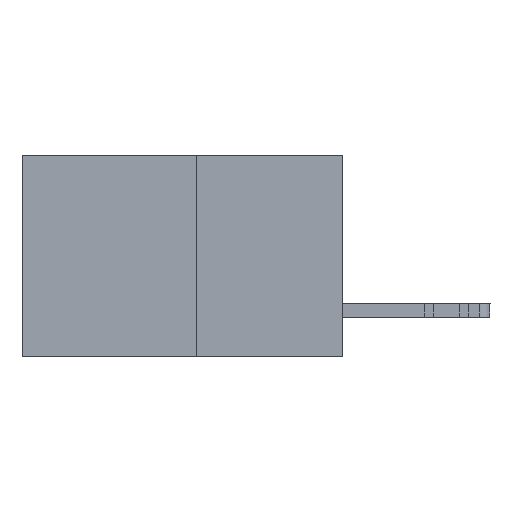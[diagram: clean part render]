
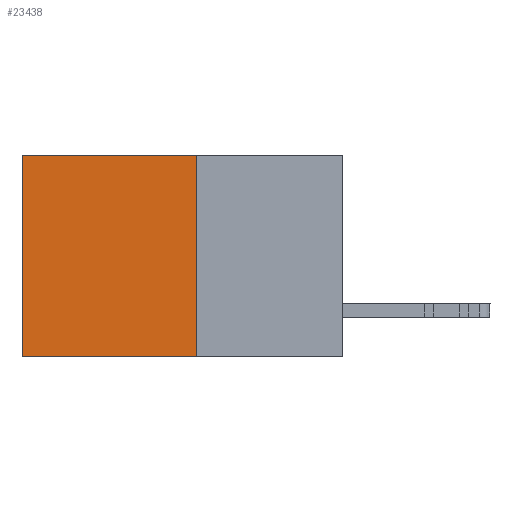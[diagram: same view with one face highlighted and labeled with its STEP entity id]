
A CAD part, left-side view. The second image highlights one B-rep face of the part: STEP entity #23438.
In plain terms, the highlighted planar face has unit normal (-1, 0, 0).
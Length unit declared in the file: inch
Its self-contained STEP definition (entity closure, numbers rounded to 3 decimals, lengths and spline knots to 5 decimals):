
#1456 = EDGE_CURVE ( 'NONE', #12765, #17585, #30709, .T. ) ;
#2441 = LINE ( 'NONE', #7972, #26798 ) ;
#4948 = PLANE ( 'NONE',  #6408 ) ;
#5959 = ORIENTED_EDGE ( 'NONE', *, *, #16981, .T. ) ;
#6408 = AXIS2_PLACEMENT_3D ( 'NONE', #10196, #27495, #12659 ) ;
#6431 = VERTEX_POINT ( 'NONE', #8429 ) ;
#7829 = ORIENTED_EDGE ( 'NONE', *, *, #24412, .F. ) ;
#7972 = CARTESIAN_POINT ( 'NONE',  ( 0.277, 0.27, -0.37 ) ) ;
#8429 = CARTESIAN_POINT ( 'NONE',  ( 0.277, 0.27, 0. ) ) ;
#9332 = CARTESIAN_POINT ( 'NONE',  ( 0.277, 0.59, -0.37 ) ) ;
#10196 = CARTESIAN_POINT ( 'NONE',  ( 0.277, 0.27, -0.37 ) ) ;
#10242 = ORIENTED_EDGE ( 'NONE', *, *, #11747, .F. ) ;
#11197 = DIRECTION ( 'NONE',  ( 0., 1., 0. ) ) ;
#11747 = EDGE_CURVE ( 'NONE', #14185, #17585, #29383, .T. ) ;
#11794 = VECTOR ( 'NONE', #29260, 39.37008 ) ;
#12659 = DIRECTION ( 'NONE',  ( 0., 0., -1. ) ) ;
#12765 = VERTEX_POINT ( 'NONE', #18227 ) ;
#13625 = CARTESIAN_POINT ( 'NONE',  ( 0.277, 0.27, -0.37 ) ) ;
#14185 = VERTEX_POINT ( 'NONE', #13625 ) ;
#16790 = VECTOR ( 'NONE', #18547, 39.37008 ) ;
#16954 = VECTOR ( 'NONE', #11197, 39.37008 ) ;
#16981 = EDGE_CURVE ( 'NONE', #6431, #12765, #31426, .T. ) ;
#17585 = VERTEX_POINT ( 'NONE', #9332 ) ;
#18227 = CARTESIAN_POINT ( 'NONE',  ( 0.277, 0.59, 0. ) ) ;
#18547 = DIRECTION ( 'NONE',  ( 0., 0., -1. ) ) ;
#18630 = CARTESIAN_POINT ( 'NONE',  ( 0.277, 0.59, -0.37 ) ) ;
#23438 = ADVANCED_FACE ( 'NONE', ( #24262 ), #4948, .F. ) ;
#24262 = FACE_OUTER_BOUND ( 'NONE', #24522, .T. ) ;
#24412 = EDGE_CURVE ( 'NONE', #6431, #14185, #2441, .T. ) ;
#24522 = EDGE_LOOP ( 'NONE', ( #25752, #10242, #7829, #5959 ) ) ;
#25752 = ORIENTED_EDGE ( 'NONE', *, *, #1456, .T. ) ;
#26769 = CARTESIAN_POINT ( 'NONE',  ( 0.277, 0.27, 0. ) ) ;
#26798 = VECTOR ( 'NONE', #27864, 39.37008 ) ;
#27495 = DIRECTION ( 'NONE',  ( 1., 0., 0. ) ) ;
#27864 = DIRECTION ( 'NONE',  ( 0., 0., -1. ) ) ;
#28488 = CARTESIAN_POINT ( 'NONE',  ( 0.277, 0.27, -0.37 ) ) ;
#29260 = DIRECTION ( 'NONE',  ( 0., 1., 0. ) ) ;
#29383 = LINE ( 'NONE', #28488, #16954 ) ;
#30709 = LINE ( 'NONE', #18630, #16790 ) ;
#31426 = LINE ( 'NONE', #26769, #11794 ) ;
